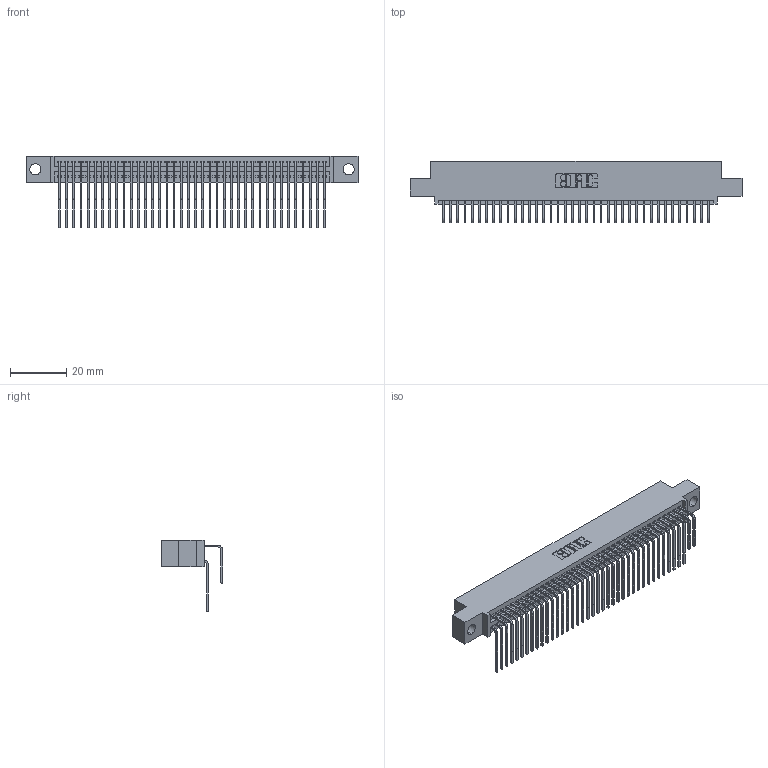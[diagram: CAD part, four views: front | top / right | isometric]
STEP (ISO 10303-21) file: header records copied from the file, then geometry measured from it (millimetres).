
FILE_DESCRIPTION (( 'STEP AP203' ), '1' );
FILE_NAME ('345-076-558-504.STEP', '2021-05-20T10:21:12', ( '' ), ( '' ), 'SwSTEP 2.0', 'SolidWorks 2020', '' );
FILE_SCHEMA (( 'CONFIG_CONTROL_DESIGN' ));
Length unit declared in the file: inch
Products named in the file (4): 345 Part_0.110 Offset - 0.156 Dia-TI; 345-292-001_558 559 Tail - 1; 345-076-558-504; 345-292-001_558 Tail - 2
Assembly tree (77 placements, depth 2):
  345-076-558-504
    345 Part_0.110 Offset - 0.156 Dia-TI
    345-292-001_558 559 Tail - 1  x38
    345-292-001_558 Tail - 2  x38
Bounding box: 117.73 x 21.83 x 25.53 mm (x, y, z)
Volume: 11658.3 mm3; surface area: 19161.5 mm2
Topology: 77 solids, 77 shells, 4096 faces, 12169 edges, 8010 vertices
Faces by surface type: plane 2758, cylinder 1338
Entity records: 32557 total; most frequent: CARTESIAN_POINT 5513, ORIENTED_EDGE 5394, DIRECTION 4837, EDGE_CURVE 2697, VECTOR 2373, LINE 2373, VERTEX_POINT 1794, AXIS2_PLACEMENT_3D 1232
